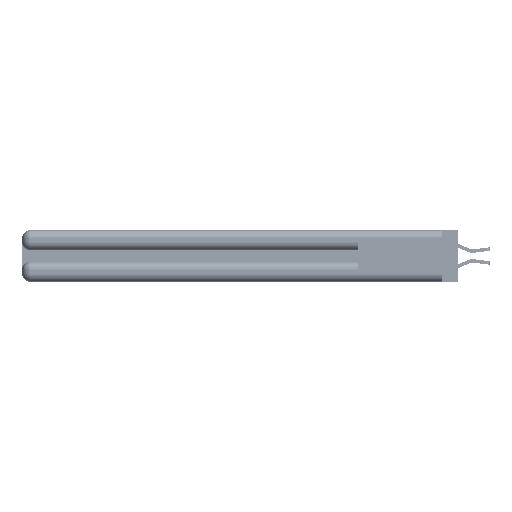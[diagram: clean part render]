
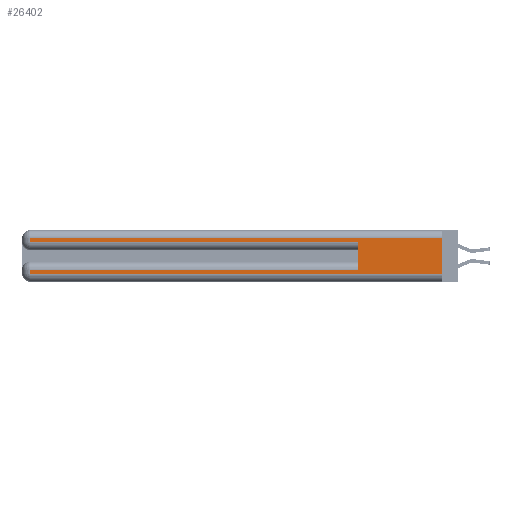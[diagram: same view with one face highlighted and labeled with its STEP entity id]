
A CAD part, left-side view. The second image highlights one B-rep face of the part: STEP entity #26402.
In plain terms, the highlighted planar face has unit normal (-1, 0, 0).
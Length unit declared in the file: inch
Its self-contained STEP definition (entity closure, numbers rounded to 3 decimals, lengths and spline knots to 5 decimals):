
#588 = VERTEX_POINT ( 'NONE', #32429 ) ;
#1160 = DIRECTION ( 'NONE',  ( 0., 0., -1. ) ) ;
#1759 = LINE ( 'NONE', #36868, #41634 ) ;
#2154 = VERTEX_POINT ( 'NONE', #30144 ) ;
#2587 = LINE ( 'NONE', #16461, #31493 ) ;
#5397 = VERTEX_POINT ( 'NONE', #34621 ) ;
#6139 = FACE_OUTER_BOUND ( 'NONE', #45389, .T. ) ;
#6306 = VECTOR ( 'NONE', #33714, 39.37008 ) ;
#6702 = ORIENTED_EDGE ( 'NONE', *, *, #9698, .T. ) ;
#7210 = LINE ( 'NONE', #45862, #26204 ) ;
#7730 = EDGE_CURVE ( 'NONE', #44112, #588, #1759, .T. ) ;
#7925 = DIRECTION ( 'NONE',  ( 0., 0., -1. ) ) ;
#8606 = DIRECTION ( 'NONE',  ( 0., -1., 0. ) ) ;
#8705 = VECTOR ( 'NONE', #22350, 39.37008 ) ;
#8951 = LINE ( 'NONE', #15436, #27931 ) ;
#9698 = EDGE_CURVE ( 'NONE', #19261, #28132, #38684, .T. ) ;
#10710 = VECTOR ( 'NONE', #29432, 39.37008 ) ;
#13417 = AXIS2_PLACEMENT_3D ( 'NONE', #45967, #23846, #1160 ) ;
#13737 = EDGE_CURVE ( 'NONE', #45935, #2154, #7210, .T. ) ;
#14101 = EDGE_CURVE ( 'NONE', #588, #45935, #30828, .T. ) ;
#14242 = CARTESIAN_POINT ( 'NONE',  ( 0., 2.94, 0.285 ) ) ;
#15436 = CARTESIAN_POINT ( 'NONE',  ( 0., 0., 0.37 ) ) ;
#16461 = CARTESIAN_POINT ( 'NONE',  ( 0., 0., 0.31 ) ) ;
#18345 = ORIENTED_EDGE ( 'NONE', *, *, #18971, .T. ) ;
#18971 = EDGE_CURVE ( 'NONE', #38004, #5397, #2587, .T. ) ;
#19261 = VERTEX_POINT ( 'NONE', #14242 ) ;
#20059 = PLANE ( 'NONE',  #13417 ) ;
#22350 = DIRECTION ( 'NONE',  ( 0., -1., 0. ) ) ;
#23846 = DIRECTION ( 'NONE',  ( 1., 0., 0. ) ) ;
#24577 = ORIENTED_EDGE ( 'NONE', *, *, #28138, .F. ) ;
#25551 = EDGE_CURVE ( 'NONE', #44112, #28132, #41382, .T. ) ;
#25563 = ORIENTED_EDGE ( 'NONE', *, *, #14101, .T. ) ;
#26204 = VECTOR ( 'NONE', #8606, 39.37008 ) ;
#26315 = CARTESIAN_POINT ( 'NONE',  ( 0., 0., 0.285 ) ) ;
#26402 = ADVANCED_FACE ( 'NONE', ( #6139 ), #20059, .F. ) ;
#26717 = ORIENTED_EDGE ( 'NONE', *, *, #44751, .T. ) ;
#27314 = DIRECTION ( 'NONE',  ( 0., 1., 0. ) ) ;
#27386 = ORIENTED_EDGE ( 'NONE', *, *, #13737, .T. ) ;
#27931 = VECTOR ( 'NONE', #7925, 39.37008 ) ;
#28132 = VERTEX_POINT ( 'NONE', #34273 ) ;
#28138 = EDGE_CURVE ( 'NONE', #38004, #2154, #8951, .T. ) ;
#28265 = ORIENTED_EDGE ( 'NONE', *, *, #25551, .F. ) ;
#29432 = DIRECTION ( 'NONE',  ( 0., 0., -1. ) ) ;
#30144 = CARTESIAN_POINT ( 'NONE',  ( 0., 0., 0.06 ) ) ;
#30828 = LINE ( 'NONE', #33122, #10710 ) ;
#31493 = VECTOR ( 'NONE', #27314, 39.37008 ) ;
#31598 = VECTOR ( 'NONE', #41076, 39.37008 ) ;
#32429 = CARTESIAN_POINT ( 'NONE',  ( 0., 2.94, 0.085 ) ) ;
#33122 = CARTESIAN_POINT ( 'NONE',  ( 0., 2.94, 0.37 ) ) ;
#33681 = CARTESIAN_POINT ( 'NONE',  ( 0., 0.6, 0.145 ) ) ;
#33714 = DIRECTION ( 'NONE',  ( 0., 0., -1. ) ) ;
#34273 = CARTESIAN_POINT ( 'NONE',  ( 0., 0.6, 0.285 ) ) ;
#34621 = CARTESIAN_POINT ( 'NONE',  ( 0., 2.94, 0.31 ) ) ;
#36307 = LINE ( 'NONE', #37437, #6306 ) ;
#36868 = CARTESIAN_POINT ( 'NONE',  ( 0., 0., 0.085 ) ) ;
#37437 = CARTESIAN_POINT ( 'NONE',  ( 0., 2.94, 0.37 ) ) ;
#37660 = CARTESIAN_POINT ( 'NONE',  ( 0., 0.6, 0.085 ) ) ;
#38004 = VERTEX_POINT ( 'NONE', #45992 ) ;
#38684 = LINE ( 'NONE', #26315, #8705 ) ;
#38810 = ORIENTED_EDGE ( 'NONE', *, *, #7730, .T. ) ;
#41076 = DIRECTION ( 'NONE',  ( 0., 0., 1. ) ) ;
#41382 = LINE ( 'NONE', #33681, #31598 ) ;
#41634 = VECTOR ( 'NONE', #44067, 39.37008 ) ;
#44067 = DIRECTION ( 'NONE',  ( 0., 1., 0. ) ) ;
#44112 = VERTEX_POINT ( 'NONE', #37660 ) ;
#44751 = EDGE_CURVE ( 'NONE', #5397, #19261, #36307, .T. ) ;
#45389 = EDGE_LOOP ( 'NONE', ( #24577, #18345, #26717, #6702, #28265, #38810, #25563, #27386 ) ) ;
#45862 = CARTESIAN_POINT ( 'NONE',  ( 0., 0., 0.06 ) ) ;
#45935 = VERTEX_POINT ( 'NONE', #47716 ) ;
#45967 = CARTESIAN_POINT ( 'NONE',  ( 0., 0., 0.37 ) ) ;
#45992 = CARTESIAN_POINT ( 'NONE',  ( 0., 0., 0.31 ) ) ;
#47716 = CARTESIAN_POINT ( 'NONE',  ( 0., 2.94, 0.06 ) ) ;
